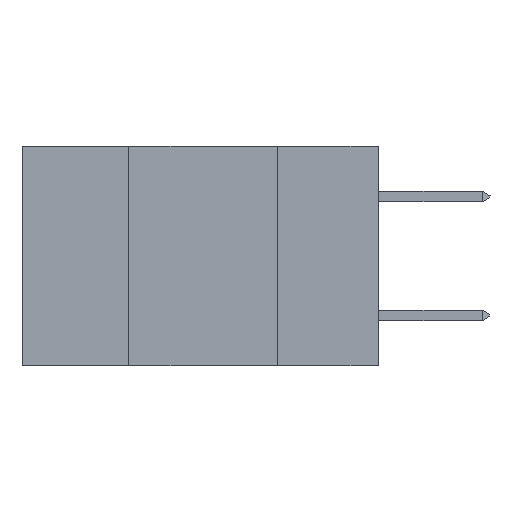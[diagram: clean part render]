
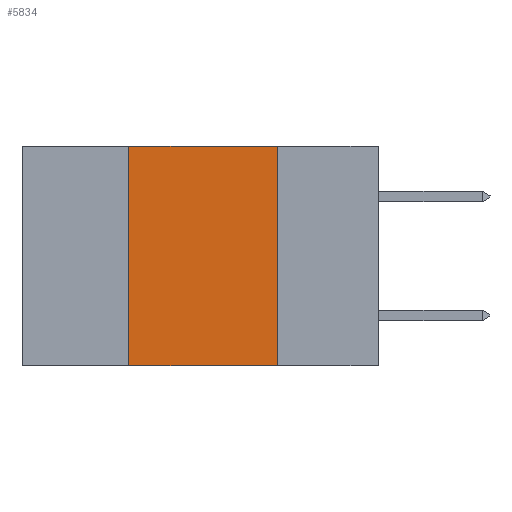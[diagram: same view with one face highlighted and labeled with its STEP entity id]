
A CAD part, left-side view. The second image highlights one B-rep face of the part: STEP entity #5834.
In plain terms, the highlighted planar face has unit normal (-1, 0, 0).
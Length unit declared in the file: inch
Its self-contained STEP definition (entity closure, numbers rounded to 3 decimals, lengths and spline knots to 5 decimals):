
#169 = DIRECTION ( 'NONE',  ( 1., 0., 0. ) ) ;
#224 = VERTEX_POINT ( 'NONE', #954 ) ;
#310 = LINE ( 'NONE', #4934, #2188 ) ;
#758 = LINE ( 'NONE', #3184, #3162 ) ;
#791 = CARTESIAN_POINT ( 'NONE',  ( 0., 0.17, 0. ) ) ;
#917 = DIRECTION ( 'NONE',  ( 0., -1., 0. ) ) ;
#925 = VECTOR ( 'NONE', #917, 39.37008 ) ;
#954 = CARTESIAN_POINT ( 'NONE',  ( 0., 0.42, 0. ) ) ;
#1158 = FACE_OUTER_BOUND ( 'NONE', #10703, .T. ) ;
#1465 = ORIENTED_EDGE ( 'NONE', *, *, #14507, .F. ) ;
#1596 = CARTESIAN_POINT ( 'NONE',  ( 0., 0.42, -0.37 ) ) ;
#2188 = VECTOR ( 'NONE', #4998, 39.37008 ) ;
#2596 = LINE ( 'NONE', #4871, #14473 ) ;
#3162 = VECTOR ( 'NONE', #10141, 39.37008 ) ;
#3184 = CARTESIAN_POINT ( 'NONE',  ( 0., 0.42, -0.37 ) ) ;
#3399 = CARTESIAN_POINT ( 'NONE',  ( 0., 0.17, -0.37 ) ) ;
#3571 = VERTEX_POINT ( 'NONE', #1596 ) ;
#4871 = CARTESIAN_POINT ( 'NONE',  ( 0., 0.17, -0.37 ) ) ;
#4934 = CARTESIAN_POINT ( 'NONE',  ( 0., 0.6, -0.37 ) ) ;
#4998 = DIRECTION ( 'NONE',  ( 0., -1., 0. ) ) ;
#5627 = PLANE ( 'NONE',  #12368 ) ;
#5834 = ADVANCED_FACE ( 'NONE', ( #1158 ), #5627, .F. ) ;
#6658 = VERTEX_POINT ( 'NONE', #3399 ) ;
#6764 = DIRECTION ( 'NONE',  ( 0., 0., -1. ) ) ;
#6916 = CARTESIAN_POINT ( 'NONE',  ( 0., 0.6, 0. ) ) ;
#8354 = DIRECTION ( 'NONE',  ( 0., 0., -1. ) ) ;
#8796 = ORIENTED_EDGE ( 'NONE', *, *, #10034, .F. ) ;
#9502 = VERTEX_POINT ( 'NONE', #791 ) ;
#9874 = EDGE_CURVE ( 'NONE', #9502, #6658, #2596, .T. ) ;
#10034 = EDGE_CURVE ( 'NONE', #224, #9502, #10460, .T. ) ;
#10141 = DIRECTION ( 'NONE',  ( 0., 0., 1. ) ) ;
#10460 = LINE ( 'NONE', #11296, #925 ) ;
#10703 = EDGE_LOOP ( 'NONE', ( #13619, #8796, #1465, #12398 ) ) ;
#11296 = CARTESIAN_POINT ( 'NONE',  ( 0., 0.6, 0. ) ) ;
#11587 = EDGE_CURVE ( 'NONE', #3571, #6658, #310, .T. ) ;
#12368 = AXIS2_PLACEMENT_3D ( 'NONE', #6916, #169, #6764 ) ;
#12398 = ORIENTED_EDGE ( 'NONE', *, *, #11587, .T. ) ;
#13619 = ORIENTED_EDGE ( 'NONE', *, *, #9874, .F. ) ;
#14473 = VECTOR ( 'NONE', #8354, 39.37008 ) ;
#14507 = EDGE_CURVE ( 'NONE', #3571, #224, #758, .T. ) ;
